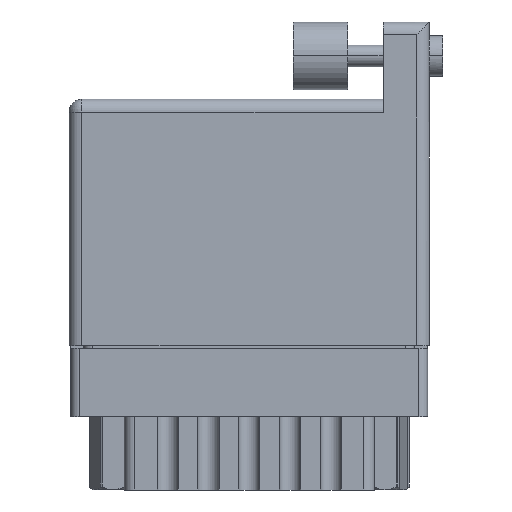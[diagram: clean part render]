
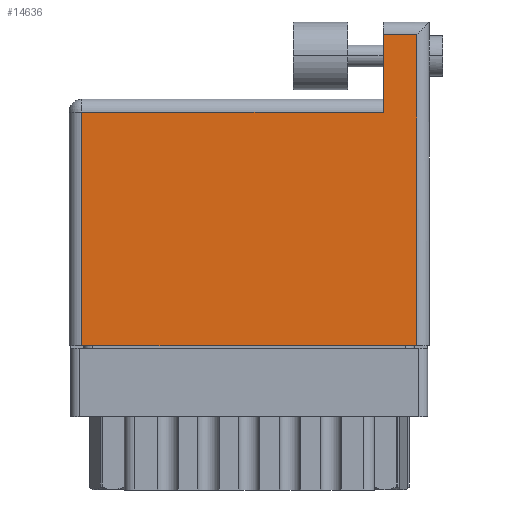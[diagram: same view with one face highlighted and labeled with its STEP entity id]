
A CAD part, front view. The second image highlights one B-rep face of the part: STEP entity #14636.
In plain terms, the highlighted face is planar.
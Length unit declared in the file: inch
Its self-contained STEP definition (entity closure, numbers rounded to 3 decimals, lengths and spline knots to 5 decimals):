
#511 = VERTEX_POINT ( 'NONE', #38879 ) ;
#1067 = CARTESIAN_POINT ( 'NONE',  ( 0., 0., 0. ) ) ;
#1069 = DIRECTION ( 'NONE',  ( 0., -1., 0. ) ) ;
#1071 = ORIENTED_EDGE ( 'NONE', *, *, #8749, .T. ) ;
#1269 = VERTEX_POINT ( 'NONE', #38547 ) ;
#1793 = ORIENTED_EDGE ( 'NONE', *, *, #32670, .T. ) ;
#3913 = LINE ( 'NONE', #37488, #5204 ) ;
#4339 = EDGE_CURVE ( 'NONE', #35639, #1269, #35848, .T. ) ;
#4433 = CARTESIAN_POINT ( 'NONE',  ( 1.155, 0.859, 0. ) ) ;
#4856 = PLANE ( 'NONE',  #33052 ) ;
#5204 = VECTOR ( 'NONE', #16030, 39.37008 ) ;
#5526 = CARTESIAN_POINT ( 'NONE',  ( 1.155, 1.143, 0. ) ) ;
#6620 = VERTEX_POINT ( 'NONE', #5526 ) ;
#7080 = VECTOR ( 'NONE', #11809, 39.37008 ) ;
#7238 = EDGE_CURVE ( 'NONE', #27983, #511, #37789, .T. ) ;
#7262 = DIRECTION ( 'NONE',  ( 0., 0., -1. ) ) ;
#8014 = EDGE_LOOP ( 'NONE', ( #1793, #22376, #22745, #1071, #14749, #33652 ) ) ;
#8117 = VERTEX_POINT ( 'NONE', #31288 ) ;
#8749 = EDGE_CURVE ( 'NONE', #6620, #35639, #13188, .T. ) ;
#9920 = CARTESIAN_POINT ( 'NONE',  ( 0.047, 0., 0. ) ) ;
#10117 = DIRECTION ( 'NONE',  ( 0., -1., 0. ) ) ;
#11809 = DIRECTION ( 'NONE',  ( -1., 0., 0. ) ) ;
#11810 = CARTESIAN_POINT ( 'NONE',  ( 1.278, 0., 0. ) ) ;
#13188 = LINE ( 'NONE', #34637, #35621 ) ;
#14046 = EDGE_CURVE ( 'NONE', #511, #6620, #3913, .T. ) ;
#14212 = LINE ( 'NONE', #9920, #16722 ) ;
#14636 = ADVANCED_FACE ( 'NONE', ( #28513 ), #4856, .F. ) ;
#14749 = ORIENTED_EDGE ( 'NONE', *, *, #4339, .T. ) ;
#16030 = DIRECTION ( 'NONE',  ( -1., 0., 0. ) ) ;
#16722 = VECTOR ( 'NONE', #10117, 39.37008 ) ;
#20102 = LINE ( 'NONE', #1067, #29384 ) ;
#22376 = ORIENTED_EDGE ( 'NONE', *, *, #7238, .T. ) ;
#22745 = ORIENTED_EDGE ( 'NONE', *, *, #14046, .T. ) ;
#25293 = DIRECTION ( 'NONE',  ( 1., 0., 0. ) ) ;
#25713 = DIRECTION ( 'NONE',  ( -1., 0., 0. ) ) ;
#26255 = DIRECTION ( 'NONE',  ( 0., 1., 0. ) ) ;
#27983 = VERTEX_POINT ( 'NONE', #11810 ) ;
#28513 = FACE_OUTER_BOUND ( 'NONE', #8014, .T. ) ;
#29384 = VECTOR ( 'NONE', #25293, 39.37008 ) ;
#31045 = CARTESIAN_POINT ( 'NONE',  ( 1.278, 1.19, 0. ) ) ;
#31288 = CARTESIAN_POINT ( 'NONE',  ( 0.047, 0., 0. ) ) ;
#31712 = VECTOR ( 'NONE', #26255, 39.37008 ) ;
#32670 = EDGE_CURVE ( 'NONE', #8117, #27983, #20102, .T. ) ;
#33052 = AXIS2_PLACEMENT_3D ( 'NONE', #38224, #7262, #25713 ) ;
#33105 = EDGE_CURVE ( 'NONE', #1269, #8117, #14212, .T. ) ;
#33440 = CARTESIAN_POINT ( 'NONE',  ( 0., 0.859, 0. ) ) ;
#33652 = ORIENTED_EDGE ( 'NONE', *, *, #33105, .T. ) ;
#34637 = CARTESIAN_POINT ( 'NONE',  ( 1.155, 1.19, 0. ) ) ;
#35621 = VECTOR ( 'NONE', #1069, 39.37008 ) ;
#35639 = VERTEX_POINT ( 'NONE', #4433 ) ;
#35848 = LINE ( 'NONE', #33440, #7080 ) ;
#37488 = CARTESIAN_POINT ( 'NONE',  ( 1.155, 1.143, 0. ) ) ;
#37789 = LINE ( 'NONE', #31045, #31712 ) ;
#38224 = CARTESIAN_POINT ( 'NONE',  ( 0., 0.906, 0. ) ) ;
#38547 = CARTESIAN_POINT ( 'NONE',  ( 0.047, 0.859, 0. ) ) ;
#38879 = CARTESIAN_POINT ( 'NONE',  ( 1.278, 1.143, 0. ) ) ;
